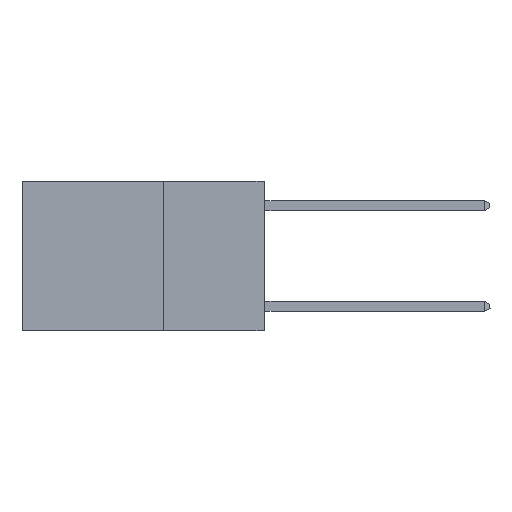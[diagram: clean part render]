
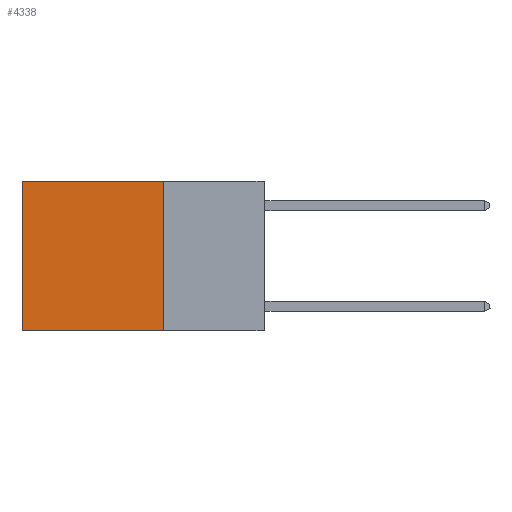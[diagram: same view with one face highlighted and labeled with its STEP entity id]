
A CAD part, left-side view. The second image highlights one B-rep face of the part: STEP entity #4338.
In plain terms, the highlighted planar face has unit normal (-1, 0, 0).
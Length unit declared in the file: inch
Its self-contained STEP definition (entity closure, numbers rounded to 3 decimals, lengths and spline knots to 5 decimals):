
#1027 = VECTOR ( 'NONE', #7379, 39.37008 ) ;
#1300 = EDGE_CURVE ( 'NONE', #6720, #4453, #2562, .T. ) ;
#1800 = ORIENTED_EDGE ( 'NONE', *, *, #6085, .T. ) ;
#1866 = CARTESIAN_POINT ( 'NONE',  ( 0.2625, 0.25, 0. ) ) ;
#1977 = VECTOR ( 'NONE', #9211, 39.37008 ) ;
#1994 = CARTESIAN_POINT ( 'NONE',  ( 0.2625, 0.25, -0.37 ) ) ;
#2038 = CARTESIAN_POINT ( 'NONE',  ( 0.2625, 0.25, 0. ) ) ;
#2436 = AXIS2_PLACEMENT_3D ( 'NONE', #9014, #6217, #10694 ) ;
#2562 = LINE ( 'NONE', #7253, #7300 ) ;
#3506 = DIRECTION ( 'NONE',  ( 0., 1., 0. ) ) ;
#4244 = ORIENTED_EDGE ( 'NONE', *, *, #1300, .F. ) ;
#4338 = ADVANCED_FACE ( 'NONE', ( #9290 ), #9865, .F. ) ;
#4453 = VERTEX_POINT ( 'NONE', #1994 ) ;
#5027 = VERTEX_POINT ( 'NONE', #6354 ) ;
#5158 = CARTESIAN_POINT ( 'NONE',  ( 0.2625, 0.6, 0. ) ) ;
#6085 = EDGE_CURVE ( 'NONE', #6720, #6955, #11470, .T. ) ;
#6217 = DIRECTION ( 'NONE',  ( 1., 0., 0. ) ) ;
#6354 = CARTESIAN_POINT ( 'NONE',  ( 0.2625, 0.6, -0.37 ) ) ;
#6368 = DIRECTION ( 'NONE',  ( 0., 0., -1. ) ) ;
#6415 = CARTESIAN_POINT ( 'NONE',  ( 0.2625, 0.6, 0. ) ) ;
#6669 = VECTOR ( 'NONE', #3506, 39.37008 ) ;
#6720 = VERTEX_POINT ( 'NONE', #2038 ) ;
#6747 = ORIENTED_EDGE ( 'NONE', *, *, #10418, .F. ) ;
#6955 = VERTEX_POINT ( 'NONE', #5158 ) ;
#7253 = CARTESIAN_POINT ( 'NONE',  ( 0.2625, 0.25, 0. ) ) ;
#7300 = VECTOR ( 'NONE', #6368, 39.37008 ) ;
#7379 = DIRECTION ( 'NONE',  ( 0., 0., -1. ) ) ;
#8194 = CARTESIAN_POINT ( 'NONE',  ( 0.2625, 0.25, -0.37 ) ) ;
#8692 = LINE ( 'NONE', #6415, #1027 ) ;
#8701 = EDGE_LOOP ( 'NONE', ( #9140, #6747, #4244, #1800 ) ) ;
#8735 = EDGE_CURVE ( 'NONE', #6955, #5027, #8692, .T. ) ;
#8809 = LINE ( 'NONE', #8194, #6669 ) ;
#9014 = CARTESIAN_POINT ( 'NONE',  ( 0.2625, 0.25, 0. ) ) ;
#9140 = ORIENTED_EDGE ( 'NONE', *, *, #8735, .T. ) ;
#9211 = DIRECTION ( 'NONE',  ( 0., 1., 0. ) ) ;
#9290 = FACE_OUTER_BOUND ( 'NONE', #8701, .T. ) ;
#9865 = PLANE ( 'NONE',  #2436 ) ;
#10418 = EDGE_CURVE ( 'NONE', #4453, #5027, #8809, .T. ) ;
#10694 = DIRECTION ( 'NONE',  ( 0., 0., -1. ) ) ;
#11470 = LINE ( 'NONE', #1866, #1977 ) ;
